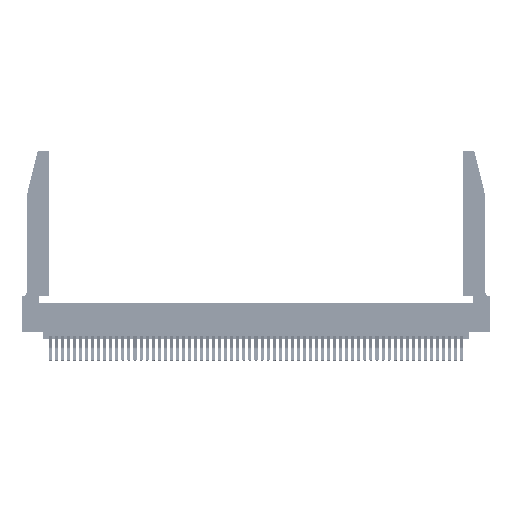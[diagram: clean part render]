
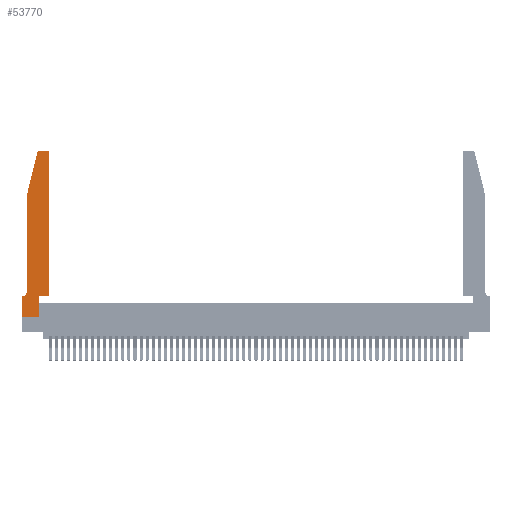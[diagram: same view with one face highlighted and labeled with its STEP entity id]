
A CAD part, top view. The second image highlights one B-rep face of the part: STEP entity #53770.
In plain terms, the highlighted planar face has unit normal (0, 0, 1).
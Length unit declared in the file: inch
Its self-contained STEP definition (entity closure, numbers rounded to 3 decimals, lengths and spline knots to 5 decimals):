
#149 = EDGE_CURVE ( 'NONE', #40581, #2930, #29234, .T. ) ;
#308 = ORIENTED_EDGE ( 'NONE', *, *, #18670, .T. ) ;
#1224 = EDGE_CURVE ( 'NONE', #2930, #17503, #43924, .T. ) ;
#1225 = DIRECTION ( 'NONE',  ( 0., 1., 0. ) ) ;
#1265 = DIRECTION ( 'NONE',  ( 0., -1., 0. ) ) ;
#1907 = DIRECTION ( 'NONE',  ( 1., 0., 0. ) ) ;
#2626 = DIRECTION ( 'NONE',  ( -1., 0., 0. ) ) ;
#2694 = CARTESIAN_POINT ( 'NONE',  ( 0.2865, 0.35, 0.37 ) ) ;
#2930 = VERTEX_POINT ( 'NONE', #47761 ) ;
#3419 = DIRECTION ( 'NONE',  ( 0., 0., 1. ) ) ;
#4311 = CARTESIAN_POINT ( 'NONE',  ( 0.284, 2.75, 0.37 ) ) ;
#4705 = CARTESIAN_POINT ( 'NONE',  ( 0.0755, 2., 0.37 ) ) ;
#5481 = EDGE_CURVE ( 'NONE', #13715, #31672, #30023, .T. ) ;
#5561 = CARTESIAN_POINT ( 'NONE',  ( 0., 0., 0.37 ) ) ;
#5786 = ORIENTED_EDGE ( 'NONE', *, *, #17107, .T. ) ;
#6672 = CARTESIAN_POINT ( 'NONE',  ( 0.0755, 2., 0.37 ) ) ;
#7274 = DIRECTION ( 'NONE',  ( 1., 0., 0. ) ) ;
#7638 = CARTESIAN_POINT ( 'NONE',  ( 0.4205, 2.75, 0.37 ) ) ;
#9030 = DIRECTION ( 'NONE',  ( -0.239, -0.971, 0. ) ) ;
#10235 = AXIS2_PLACEMENT_3D ( 'NONE', #44770, #18991, #49036 ) ;
#11106 = CARTESIAN_POINT ( 'NONE',  ( 0.0755, 0.35, 0.37 ) ) ;
#11696 = AXIS2_PLACEMENT_3D ( 'NONE', #29187, #3419, #33545 ) ;
#12105 = LINE ( 'NONE', #35607, #33658 ) ;
#12797 = AXIS2_PLACEMENT_3D ( 'NONE', #13460, #43561, #17822 ) ;
#13099 = VERTEX_POINT ( 'NONE', #7638 ) ;
#13103 = LINE ( 'NONE', #5561, #46054 ) ;
#13460 = CARTESIAN_POINT ( 'NONE',  ( 0.284, 2.72, 0.37 ) ) ;
#13715 = VERTEX_POINT ( 'NONE', #49061 ) ;
#13918 = CARTESIAN_POINT ( 'NONE',  ( 0.4505, 0.35, 0.37 ) ) ;
#15830 = ORIENTED_EDGE ( 'NONE', *, *, #29456, .T. ) ;
#16198 = FACE_OUTER_BOUND ( 'NONE', #25606, .T. ) ;
#17107 = EDGE_CURVE ( 'NONE', #17503, #21933, #37159, .T. ) ;
#17171 = ORIENTED_EDGE ( 'NONE', *, *, #5481, .T. ) ;
#17503 = VERTEX_POINT ( 'NONE', #46962 ) ;
#17822 = DIRECTION ( 'NONE',  ( 1., 0., 0. ) ) ;
#18601 = VECTOR ( 'NONE', #32799, 39.37008 ) ;
#18670 = EDGE_CURVE ( 'NONE', #46078, #13099, #20936, .T. ) ;
#18991 = DIRECTION ( 'NONE',  ( 0., 0., -1. ) ) ;
#19213 = VERTEX_POINT ( 'NONE', #32547 ) ;
#19837 = LINE ( 'NONE', #52635, #41357 ) ;
#20936 = CIRCLE ( 'NONE', #11696, 0.03 ) ;
#21933 = VERTEX_POINT ( 'NONE', #44625 ) ;
#22871 = EDGE_CURVE ( 'NONE', #13099, #26975, #12105, .T. ) ;
#23344 = CARTESIAN_POINT ( 'NONE',  ( 0., 0.35, 0.37 ) ) ;
#25357 = CIRCLE ( 'NONE', #12797, 0.03 ) ;
#25558 = VECTOR ( 'NONE', #39886, 39.37008 ) ;
#25606 = EDGE_LOOP ( 'NONE', ( #55294, #50263, #25780, #48661, #5786, #25790, #26439, #45228, #17171, #54503, #15830, #308 ) ) ;
#25780 = ORIENTED_EDGE ( 'NONE', *, *, #149, .T. ) ;
#25790 = ORIENTED_EDGE ( 'NONE', *, *, #53879, .T. ) ;
#26439 = ORIENTED_EDGE ( 'NONE', *, *, #50673, .T. ) ;
#26518 = VECTOR ( 'NONE', #7274, 39.37008 ) ;
#26975 = VERTEX_POINT ( 'NONE', #4311 ) ;
#27372 = VERTEX_POINT ( 'NONE', #29074 ) ;
#27661 = DIRECTION ( 'NONE',  ( 0., 0., 1. ) ) ;
#29074 = CARTESIAN_POINT ( 'NONE',  ( 0., 0., 0.37 ) ) ;
#29187 = CARTESIAN_POINT ( 'NONE',  ( 0.4205, 2.72, 0.37 ) ) ;
#29234 = LINE ( 'NONE', #4705, #40685 ) ;
#29456 = EDGE_CURVE ( 'NONE', #19213, #46078, #19837, .T. ) ;
#29529 = CARTESIAN_POINT ( 'NONE',  ( 0., 0.35, 0.37 ) ) ;
#30023 = LINE ( 'NONE', #2694, #18601 ) ;
#30432 = EDGE_CURVE ( 'NONE', #27372, #13715, #49371, .T. ) ;
#31021 = CARTESIAN_POINT ( 'NONE',  ( 0.2865, 0.35, 0.37 ) ) ;
#31672 = VERTEX_POINT ( 'NONE', #31021 ) ;
#32547 = CARTESIAN_POINT ( 'NONE',  ( 0.4505, 0.35, 0.37 ) ) ;
#32799 = DIRECTION ( 'NONE',  ( 0., 1., 0. ) ) ;
#33545 = DIRECTION ( 'NONE',  ( 1., 0., 0. ) ) ;
#33658 = VECTOR ( 'NONE', #39932, 39.37008 ) ;
#35607 = CARTESIAN_POINT ( 'NONE',  ( 0.2605, 2.75, 0.37 ) ) ;
#37009 = LINE ( 'NONE', #13918, #25558 ) ;
#37159 = CIRCLE ( 'NONE', #10235, 0.07 ) ;
#37399 = CARTESIAN_POINT ( 'NONE',  ( 0., 0., 0.37 ) ) ;
#38698 = VERTEX_POINT ( 'NONE', #29529 ) ;
#39886 = DIRECTION ( 'NONE',  ( 1., 0., 0. ) ) ;
#39932 = DIRECTION ( 'NONE',  ( -1., 0., 0. ) ) ;
#39954 = CARTESIAN_POINT ( 'NONE',  ( 0.4505, 2.72, 0.37 ) ) ;
#40581 = VERTEX_POINT ( 'NONE', #43251 ) ;
#40685 = VECTOR ( 'NONE', #9030, 39.37008 ) ;
#40713 = VECTOR ( 'NONE', #2626, 39.37008 ) ;
#41086 = DIRECTION ( 'NONE',  ( 0., -1., 0. ) ) ;
#41357 = VECTOR ( 'NONE', #1225, 39.37008 ) ;
#42858 = EDGE_CURVE ( 'NONE', #31672, #19213, #37009, .T. ) ;
#43251 = CARTESIAN_POINT ( 'NONE',  ( 0.25487, 2.72718, 0.37 ) ) ;
#43561 = DIRECTION ( 'NONE',  ( 0., 0., 1. ) ) ;
#43924 = LINE ( 'NONE', #6672, #53863 ) ;
#44565 = AXIS2_PLACEMENT_3D ( 'NONE', #23344, #27661, #1907 ) ;
#44625 = CARTESIAN_POINT ( 'NONE',  ( 0.0055, 0.35, 0.37 ) ) ;
#44770 = CARTESIAN_POINT ( 'NONE',  ( 0.0055, 0.42, 0.37 ) ) ;
#45228 = ORIENTED_EDGE ( 'NONE', *, *, #30432, .T. ) ;
#45423 = EDGE_CURVE ( 'NONE', #26975, #40581, #25357, .T. ) ;
#46054 = VECTOR ( 'NONE', #1265, 39.37008 ) ;
#46078 = VERTEX_POINT ( 'NONE', #39954 ) ;
#46962 = CARTESIAN_POINT ( 'NONE',  ( 0.0755, 0.42, 0.37 ) ) ;
#47761 = CARTESIAN_POINT ( 'NONE',  ( 0.0755, 2., 0.37 ) ) ;
#48661 = ORIENTED_EDGE ( 'NONE', *, *, #1224, .T. ) ;
#49036 = DIRECTION ( 'NONE',  ( -1., 0., 0. ) ) ;
#49054 = PLANE ( 'NONE',  #44565 ) ;
#49061 = CARTESIAN_POINT ( 'NONE',  ( 0.2865, 0., 0.37 ) ) ;
#49371 = LINE ( 'NONE', #37399, #26518 ) ;
#50263 = ORIENTED_EDGE ( 'NONE', *, *, #45423, .T. ) ;
#50673 = EDGE_CURVE ( 'NONE', #38698, #27372, #13103, .T. ) ;
#52070 = LINE ( 'NONE', #11106, #40713 ) ;
#52635 = CARTESIAN_POINT ( 'NONE',  ( 0.4505, 0.35, 0.37 ) ) ;
#53770 = ADVANCED_FACE ( 'NONE', ( #16198 ), #49054, .T. ) ;
#53863 = VECTOR ( 'NONE', #41086, 39.37008 ) ;
#53879 = EDGE_CURVE ( 'NONE', #21933, #38698, #52070, .T. ) ;
#54503 = ORIENTED_EDGE ( 'NONE', *, *, #42858, .T. ) ;
#55294 = ORIENTED_EDGE ( 'NONE', *, *, #22871, .T. ) ;
